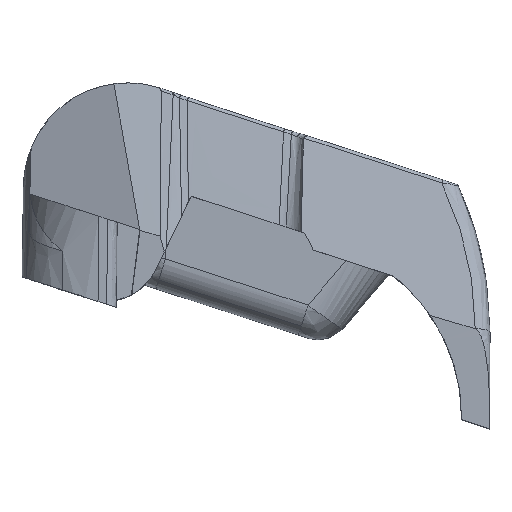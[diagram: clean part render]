
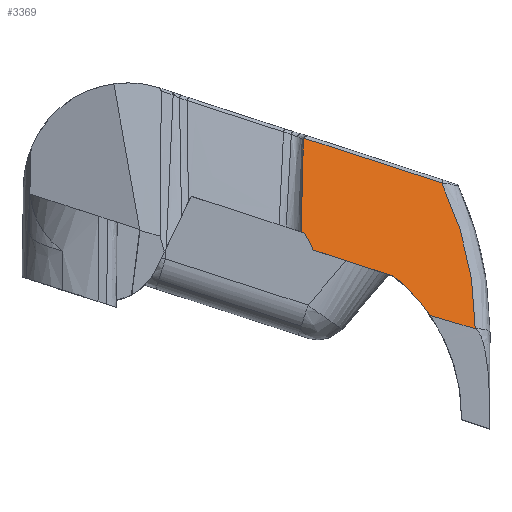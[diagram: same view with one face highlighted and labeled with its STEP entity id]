
A CAD part, top view. The second image highlights one B-rep face of the part: STEP entity #3369.
In plain terms, the highlighted free-form (B-spline) face has degree [3, 3] with [4, 4] control points.
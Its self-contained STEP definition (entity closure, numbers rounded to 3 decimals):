
#41 = LINE ( 'NONE', #5342, #2814 ) ;
#92 = FACE_OUTER_BOUND ( 'NONE', #1519, .T. ) ;
#108 = B_SPLINE_CURVE_WITH_KNOTS ( 'NONE', 3,
 ( #326, #582, #1557, #4911 ),
 .UNSPECIFIED., .F., .F.,
 ( 4, 4 ),
 ( 0., 1. ),
 .UNSPECIFIED. ) ;
#294 = CARTESIAN_POINT ( 'NONE',  ( 13.985, 54.676, 4.503 ) ) ;
#325 = CARTESIAN_POINT ( 'NONE',  ( 11.287, 46.725, 6.238 ) ) ;
#326 = CARTESIAN_POINT ( 'NONE',  ( 12.019, 55.314, 4.503 ) ) ;
#342 = VERTEX_POINT ( 'NONE', #1628 ) ;
#362 = EDGE_CURVE ( 'NONE', #1514, #731, #5002, .T. ) ;
#474 = VERTEX_POINT ( 'NONE', #635 ) ;
#488 = CARTESIAN_POINT ( 'NONE',  ( 9.548, 48.771, 5.938 ) ) ;
#582 = CARTESIAN_POINT ( 'NONE',  ( 13.448, 52.371, 4.992 ) ) ;
#592 = CARTESIAN_POINT ( 'NONE',  ( 12.702, 46.308, 6.238 ) ) ;
#635 = CARTESIAN_POINT ( 'NONE',  ( 3.16, 52.063, 5.674 ) ) ;
#637 = B_SPLINE_CURVE_WITH_KNOTS ( 'NONE', 3,
 ( #3871, #488, #1453, #4817, #1949, #5280 ),
 .UNSPECIFIED., .F., .F.,
 ( 4, 2, 4 ),
 ( -1.088, -0.847, -0.737 ),
 .UNSPECIFIED. ) ;
#731 = VERTEX_POINT ( 'NONE', #5969 ) ;
#756 = CARTESIAN_POINT ( 'NONE',  ( 3.71, 50.963, 5.853 ) ) ;
#772 = CARTESIAN_POINT ( 'NONE',  ( 12.991, 49.114, 5.667 ) ) ;
#1027 = VERTEX_POINT ( 'NONE', #2186 ) ;
#1058 = CARTESIAN_POINT ( 'NONE',  ( 3.066, 58.093, 4.526 ) ) ;
#1073 = CARTESIAN_POINT ( 'NONE',  ( 14.002, 45.924, 6.238 ) ) ;
#1098 = VERTEX_POINT ( 'NONE', #6127 ) ;
#1254 = CARTESIAN_POINT ( 'NONE',  ( 12.81, 55.057, 4.503 ) ) ;
#1308 = CARTESIAN_POINT ( 'NONE',  ( 9.045, 56.28, 4.503 ) ) ;
#1390 = B_SPLINE_CURVE_WITH_KNOTS ( 'NONE', 3,
 ( #3739, #4212, #1308, #4695 ),
 .UNSPECIFIED., .F., .F.,
 ( 4, 4 ),
 ( -0.938, 0. ),
 .UNSPECIFIED. ) ;
#1453 = CARTESIAN_POINT ( 'NONE',  ( 10.121, 48.209, 6.015 ) ) ;
#1503 = CARTESIAN_POINT ( 'NONE',  ( 12.019, 55.314, 4.503 ) ) ;
#1514 = VERTEX_POINT ( 'NONE', #3662 ) ;
#1519 = EDGE_LOOP ( 'NONE', ( #3226, #3361, #1785, #5577, #5712, #4643, #1986, #5771, #2151 ) ) ;
#1557 = CARTESIAN_POINT ( 'NONE',  ( 14.189, 49.116, 5.594 ) ) ;
#1590 = EDGE_CURVE ( 'NONE', #731, #2482, #1390, .T. ) ;
#1628 = CARTESIAN_POINT ( 'NONE',  ( 14.187, 45.869, 6.238 ) ) ;
#1712 = CARTESIAN_POINT ( 'NONE',  ( 3.71, 50.963, 5.853 ) ) ;
#1741 = EDGE_CURVE ( 'NONE', #1027, #1514, #41, .T. ) ;
#1761 = CARTESIAN_POINT ( 'NONE',  ( 6.488, 51.227, 5.64 ) ) ;
#1785 = ORIENTED_EDGE ( 'NONE', *, *, #1741, .F. ) ;
#1949 = CARTESIAN_POINT ( 'NONE',  ( 11.082, 47.024, 6.191 ) ) ;
#1986 = ORIENTED_EDGE ( 'NONE', *, *, #3867, .T. ) ;
#1998 = VECTOR ( 'NONE', #3747, 1000. ) ;
#2151 = ORIENTED_EDGE ( 'NONE', *, *, #3201, .F. ) ;
#2186 = CARTESIAN_POINT ( 'NONE',  ( 2.923, 52.14, 5.673 ) ) ;
#2197 = B_SPLINE_SURFACE_WITH_KNOTS ( 'NONE', 3, 3, ( 
 ( #4223, #6023, #3199, #294 ),
 ( #3684, #772, #4159, #1254 ),
 ( #4644, #1761, #5114, #2249 ),
 ( #5563, #2743, #6055, #3228 ) ),
 .UNSPECIFIED., .F., .F., .F.,
 ( 4, 4 ),
 ( 4, 4 ),
 ( 0.06, 1. ),
 ( 0.402, 0.986 ),
 .UNSPECIFIED. ) ;
#2204 = CARTESIAN_POINT ( 'NONE',  ( 7.154, 49.844, 5.869 ) ) ;
#2249 = CARTESIAN_POINT ( 'NONE',  ( 6.54, 57.095, 4.502 ) ) ;
#2283 = EDGE_CURVE ( 'NONE', #3813, #342, #5253, .T. ) ;
#2478 = CARTESIAN_POINT ( 'NONE',  ( 3.078, 58.176, 4.51 ) ) ;
#2482 = VERTEX_POINT ( 'NONE', #1503 ) ;
#2500 = DIRECTION ( 'NONE',  ( 0.024, 0.982, -0.189 ) ) ;
#2666 = CARTESIAN_POINT ( 'NONE',  ( 3.343, 51.696, 5.733 ) ) ;
#2743 = CARTESIAN_POINT ( 'NONE',  ( 2.929, 52.383, 5.626 ) ) ;
#2814 = VECTOR ( 'NONE', #2500, 1000. ) ;
#3004 = EDGE_CURVE ( 'NONE', #1027, #474, #3319, .T. ) ;
#3199 = CARTESIAN_POINT ( 'NONE',  ( 14.06, 51.709, 5.087 ) ) ;
#3201 = EDGE_CURVE ( 'NONE', #2482, #342, #108, .T. ) ;
#3226 = ORIENTED_EDGE ( 'NONE', *, *, #1590, .F. ) ;
#3228 = CARTESIAN_POINT ( 'NONE',  ( 3.069, 58.222, 4.502 ) ) ;
#3264 = CARTESIAN_POINT ( 'NONE',  ( 3.04, 52.102, 5.673 ) ) ;
#3319 = LINE ( 'NONE', #3264, #1998 ) ;
#3361 = ORIENTED_EDGE ( 'NONE', *, *, #362, .F. ) ;
#3369 = ADVANCED_FACE ( 'NONE', ( #92 ), #2197, .F. ) ;
#3662 = CARTESIAN_POINT ( 'NONE',  ( 3.066, 58.093, 4.526 ) ) ;
#3666 = CARTESIAN_POINT ( 'NONE',  ( 3.527, 51.329, 5.793 ) ) ;
#3684 = CARTESIAN_POINT ( 'NONE',  ( 13.081, 46.142, 6.249 ) ) ;
#3731 = EDGE_CURVE ( 'NONE', #1098, #5576, #4005, .T. ) ;
#3739 = CARTESIAN_POINT ( 'NONE',  ( 3.098, 58.211, 4.502 ) ) ;
#3747 = DIRECTION ( 'NONE',  ( 0.951, -0.309, 0.004 ) ) ;
#3813 = VERTEX_POINT ( 'NONE', #325 ) ;
#3867 = EDGE_CURVE ( 'NONE', #5576, #3813, #637, .T. ) ;
#3871 = CARTESIAN_POINT ( 'NONE',  ( 8.921, 49.27, 5.878 ) ) ;
#3973 = CARTESIAN_POINT ( 'NONE',  ( 13.671, 46.022, 6.238 ) ) ;
#4001 = CARTESIAN_POINT ( 'NONE',  ( 3.066, 58.136, 4.518 ) ) ;
#4005 = B_SPLINE_CURVE_WITH_KNOTS ( 'NONE', 3,
 ( #1712, #4599, #2204, #5520 ),
 .UNSPECIFIED., .F., .F.,
 ( 4, 4 ),
 ( -0.612, -0.05 ),
 .UNSPECIFIED. ) ;
#4159 = CARTESIAN_POINT ( 'NONE',  ( 12.901, 52.085, 5.085 ) ) ;
#4212 = CARTESIAN_POINT ( 'NONE',  ( 6.072, 57.246, 4.502 ) ) ;
#4223 = CARTESIAN_POINT ( 'NONE',  ( 14.21, 45.775, 6.256 ) ) ;
#4461 = CARTESIAN_POINT ( 'NONE',  ( 14.187, 45.869, 6.238 ) ) ;
#4599 = CARTESIAN_POINT ( 'NONE',  ( 5.252, 50.462, 5.86 ) ) ;
#4643 = ORIENTED_EDGE ( 'NONE', *, *, #3731, .T. ) ;
#4644 = CARTESIAN_POINT ( 'NONE',  ( 6.461, 48.293, 6.209 ) ) ;
#4695 = CARTESIAN_POINT ( 'NONE',  ( 12.019, 55.314, 4.503 ) ) ;
#4817 = CARTESIAN_POINT ( 'NONE',  ( 10.864, 47.315, 6.147 ) ) ;
#4911 = CARTESIAN_POINT ( 'NONE',  ( 14.187, 45.869, 6.238 ) ) ;
#4927 = EDGE_CURVE ( 'NONE', #474, #1098, #5476, .T. ) ;
#5002 = B_SPLINE_CURVE_WITH_KNOTS ( 'NONE', 3,
 ( #1058, #4001, #2478, #5316 ),
 .UNSPECIFIED., .F., .F.,
 ( 4, 4 ),
 ( 0., 1. ),
 .UNSPECIFIED. ) ;
#5114 = CARTESIAN_POINT ( 'NONE',  ( 6.514, 54.161, 5.071 ) ) ;
#5253 = B_SPLINE_CURVE_WITH_KNOTS ( 'NONE', 3,
 ( #5826, #5364, #592, #3973, #1073, #4461 ),
 .UNSPECIFIED., .F., .F.,
 ( 4, 2, 4 ),
 ( 0., 0.5, 1. ),
 .UNSPECIFIED. ) ;
#5280 = CARTESIAN_POINT ( 'NONE',  ( 11.287, 46.725, 6.238 ) ) ;
#5314 = CARTESIAN_POINT ( 'NONE',  ( 8.921, 49.27, 5.878 ) ) ;
#5316 = CARTESIAN_POINT ( 'NONE',  ( 3.098, 58.211, 4.502 ) ) ;
#5342 = CARTESIAN_POINT ( 'NONE',  ( 2.713, 43.435, 7.349 ) ) ;
#5364 = CARTESIAN_POINT ( 'NONE',  ( 12.063, 46.496, 6.238 ) ) ;
#5476 = B_SPLINE_CURVE_WITH_KNOTS ( 'NONE', 3,
 ( #6004, #2666, #3666, #756 ),
 .UNSPECIFIED., .F., .F.,
 ( 4, 4 ),
 ( -0.175, -0.051 ),
 .UNSPECIFIED. ) ;
#5520 = CARTESIAN_POINT ( 'NONE',  ( 8.921, 49.27, 5.878 ) ) ;
#5563 = CARTESIAN_POINT ( 'NONE',  ( 2.858, 49.463, 6.188 ) ) ;
#5576 = VERTEX_POINT ( 'NONE', #5314 ) ;
#5577 = ORIENTED_EDGE ( 'NONE', *, *, #3004, .T. ) ;
#5712 = ORIENTED_EDGE ( 'NONE', *, *, #4927, .T. ) ;
#5771 = ORIENTED_EDGE ( 'NONE', *, *, #2283, .T. ) ;
#5826 = CARTESIAN_POINT ( 'NONE',  ( 11.287, 46.725, 6.238 ) ) ;
#5969 = CARTESIAN_POINT ( 'NONE',  ( 3.098, 58.211, 4.502 ) ) ;
#6004 = CARTESIAN_POINT ( 'NONE',  ( 3.16, 52.063, 5.674 ) ) ;
#6023 = CARTESIAN_POINT ( 'NONE',  ( 14.135, 48.742, 5.671 ) ) ;
#6055 = CARTESIAN_POINT ( 'NONE',  ( 2.999, 55.303, 5.064 ) ) ;
#6127 = CARTESIAN_POINT ( 'NONE',  ( 3.71, 50.963, 5.853 ) ) ;
